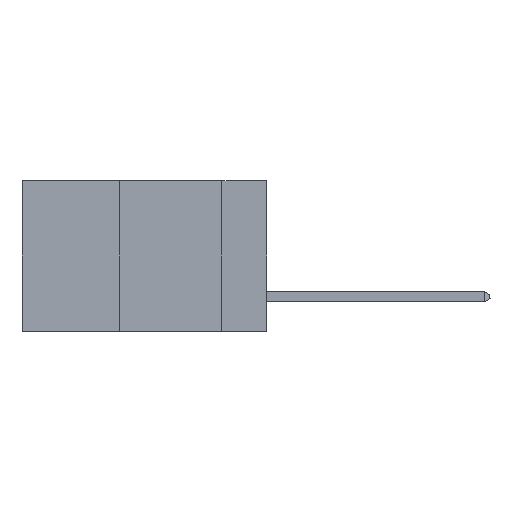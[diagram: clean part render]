
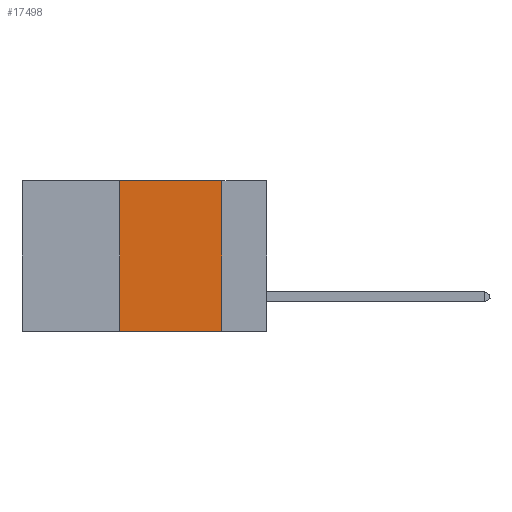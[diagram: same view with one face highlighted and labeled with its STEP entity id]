
A CAD part, left-side view. The second image highlights one B-rep face of the part: STEP entity #17498.
In plain terms, the highlighted planar face has unit normal (-1, 0, 0).
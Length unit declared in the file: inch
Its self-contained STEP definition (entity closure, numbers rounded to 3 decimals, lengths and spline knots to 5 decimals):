
#444 = ORIENTED_EDGE ( 'NONE', *, *, #6017, .F. ) ;
#529 = DIRECTION ( 'NONE',  ( 0., -1., 0. ) ) ;
#2709 = DIRECTION ( 'NONE',  ( 0., 0., -1. ) ) ;
#4308 = LINE ( 'NONE', #19216, #37917 ) ;
#4662 = VECTOR ( 'NONE', #5444, 39.37008 ) ;
#5444 = DIRECTION ( 'NONE',  ( 0., 0., -1. ) ) ;
#6017 = EDGE_CURVE ( 'NONE', #16035, #11492, #14945, .T. ) ;
#6613 = VECTOR ( 'NONE', #27687, 39.37008 ) ;
#8723 = PLANE ( 'NONE',  #11030 ) ;
#9050 = ORIENTED_EDGE ( 'NONE', *, *, #38403, .F. ) ;
#9060 = CARTESIAN_POINT ( 'NONE',  ( 0., 0.36, -0.37 ) ) ;
#9246 = ORIENTED_EDGE ( 'NONE', *, *, #18776, .T. ) ;
#11030 = AXIS2_PLACEMENT_3D ( 'NONE', #18128, #17984, #2709 ) ;
#11492 = VERTEX_POINT ( 'NONE', #14194 ) ;
#12617 = ORIENTED_EDGE ( 'NONE', *, *, #13878, .F. ) ;
#12757 = FACE_OUTER_BOUND ( 'NONE', #20301, .T. ) ;
#13878 = EDGE_CURVE ( 'NONE', #21782, #29536, #35409, .T. ) ;
#14194 = CARTESIAN_POINT ( 'NONE',  ( 0., 0.36, 0. ) ) ;
#14945 = LINE ( 'NONE', #23337, #6613 ) ;
#16035 = VERTEX_POINT ( 'NONE', #9060 ) ;
#17498 = ADVANCED_FACE ( 'NONE', ( #12757 ), #8723, .F. ) ;
#17984 = DIRECTION ( 'NONE',  ( 1., 0., 0. ) ) ;
#18128 = CARTESIAN_POINT ( 'NONE',  ( 0., 0.6, 0. ) ) ;
#18776 = EDGE_CURVE ( 'NONE', #16035, #29536, #4308, .T. ) ;
#19216 = CARTESIAN_POINT ( 'NONE',  ( 0., 0.6, -0.37 ) ) ;
#20301 = EDGE_LOOP ( 'NONE', ( #12617, #9050, #444, #9246 ) ) ;
#21782 = VERTEX_POINT ( 'NONE', #30219 ) ;
#23337 = CARTESIAN_POINT ( 'NONE',  ( 0., 0.36, 0. ) ) ;
#23450 = VECTOR ( 'NONE', #27663, 39.37008 ) ;
#27663 = DIRECTION ( 'NONE',  ( 0., -1., 0. ) ) ;
#27687 = DIRECTION ( 'NONE',  ( 0., 0., 1. ) ) ;
#29536 = VERTEX_POINT ( 'NONE', #36949 ) ;
#30219 = CARTESIAN_POINT ( 'NONE',  ( 0., 0.11, 0. ) ) ;
#31269 = CARTESIAN_POINT ( 'NONE',  ( 0., 0.6, 0. ) ) ;
#31285 = LINE ( 'NONE', #31269, #23450 ) ;
#35409 = LINE ( 'NONE', #35993, #4662 ) ;
#35993 = CARTESIAN_POINT ( 'NONE',  ( 0., 0.11, 0. ) ) ;
#36949 = CARTESIAN_POINT ( 'NONE',  ( 0., 0.11, -0.37 ) ) ;
#37917 = VECTOR ( 'NONE', #529, 39.37008 ) ;
#38403 = EDGE_CURVE ( 'NONE', #11492, #21782, #31285, .T. ) ;
